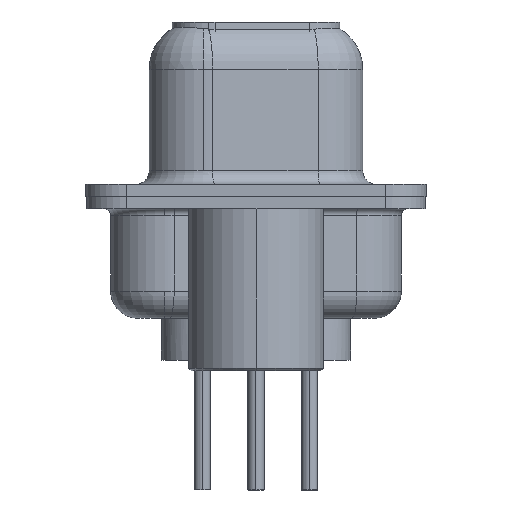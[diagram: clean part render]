
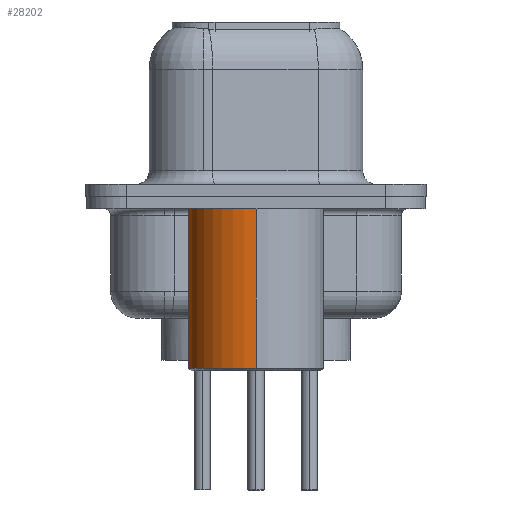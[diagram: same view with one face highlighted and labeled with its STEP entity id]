
A CAD part, left-side view. The second image highlights one B-rep face of the part: STEP entity #28202.
In plain terms, the highlighted cylindrical face has radius 2.5 mm (diameter 5 mm), a partial arc.
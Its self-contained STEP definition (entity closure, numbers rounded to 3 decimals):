
#35 = DIRECTION ( 'NONE',  ( 1., 0., 0. ) ) ;
#229 = VERTEX_POINT ( 'NONE', #9775 ) ;
#1061 = ORIENTED_EDGE ( 'NONE', *, *, #17779, .F. ) ;
#2935 = CIRCLE ( 'NONE', #14210, 2.5 ) ;
#3417 = VERTEX_POINT ( 'NONE', #5167 ) ;
#3421 = DIRECTION ( 'NONE',  ( 0., 0., 1. ) ) ;
#5167 = CARTESIAN_POINT ( 'NONE',  ( -2.5, 0., -6.35 ) ) ;
#5636 = LINE ( 'NONE', #21242, #21952 ) ;
#6053 = LINE ( 'NONE', #10490, #19998 ) ;
#6708 = VERTEX_POINT ( 'NONE', #22396 ) ;
#7572 = ORIENTED_EDGE ( 'NONE', *, *, #8138, .T. ) ;
#8138 = EDGE_CURVE ( 'NONE', #3417, #229, #6053, .T. ) ;
#8455 = EDGE_LOOP ( 'NONE', ( #17094, #7572, #1061, #26217 ) ) ;
#8886 = DIRECTION ( 'NONE',  ( 0., 0., 1. ) ) ;
#9418 = DIRECTION ( 'NONE',  ( 1., 0., 0. ) ) ;
#9775 = CARTESIAN_POINT ( 'NONE',  ( -2.5, 0., -0.45 ) ) ;
#10279 = CARTESIAN_POINT ( 'NONE',  ( 0., 0., -6.35 ) ) ;
#10417 = EDGE_CURVE ( 'NONE', #6708, #19327, #5636, .T. ) ;
#10424 = DIRECTION ( 'NONE',  ( 0., 0., 1. ) ) ;
#10490 = CARTESIAN_POINT ( 'NONE',  ( -2.5, 0., 0.581 ) ) ;
#11176 = CARTESIAN_POINT ( 'NONE',  ( 0., 0., 0.581 ) ) ;
#11611 = FACE_OUTER_BOUND ( 'NONE', #8455, .T. ) ;
#12865 = EDGE_CURVE ( 'NONE', #6708, #3417, #27200, .T. ) ;
#13422 = CARTESIAN_POINT ( 'NONE',  ( 0., 0., -0.45 ) ) ;
#13655 = AXIS2_PLACEMENT_3D ( 'NONE', #11176, #25892, #9418 ) ;
#14210 = AXIS2_PLACEMENT_3D ( 'NONE', #13422, #8886, #35 ) ;
#15752 = CARTESIAN_POINT ( 'NONE',  ( 2.5, 0., -0.45 ) ) ;
#16874 = DIRECTION ( 'NONE',  ( 1., 0., 0. ) ) ;
#17094 = ORIENTED_EDGE ( 'NONE', *, *, #12865, .T. ) ;
#17779 = EDGE_CURVE ( 'NONE', #19327, #229, #2935, .T. ) ;
#19327 = VERTEX_POINT ( 'NONE', #15752 ) ;
#19998 = VECTOR ( 'NONE', #21787, 1000. ) ;
#21242 = CARTESIAN_POINT ( 'NONE',  ( 2.5, 0., 0.581 ) ) ;
#21787 = DIRECTION ( 'NONE',  ( 0., 0., 1. ) ) ;
#21952 = VECTOR ( 'NONE', #3421, 1000. ) ;
#22396 = CARTESIAN_POINT ( 'NONE',  ( 2.5, 0., -6.35 ) ) ;
#22921 = CYLINDRICAL_SURFACE ( 'NONE', #13655, 2.5 ) ;
#25808 = AXIS2_PLACEMENT_3D ( 'NONE', #10279, #10424, #16874 ) ;
#25892 = DIRECTION ( 'NONE',  ( 0., 0., 1. ) ) ;
#26217 = ORIENTED_EDGE ( 'NONE', *, *, #10417, .F. ) ;
#27200 = CIRCLE ( 'NONE', #25808, 2.5 ) ;
#28202 = ADVANCED_FACE ( 'NONE', ( #11611 ), #22921, .T. ) ;
